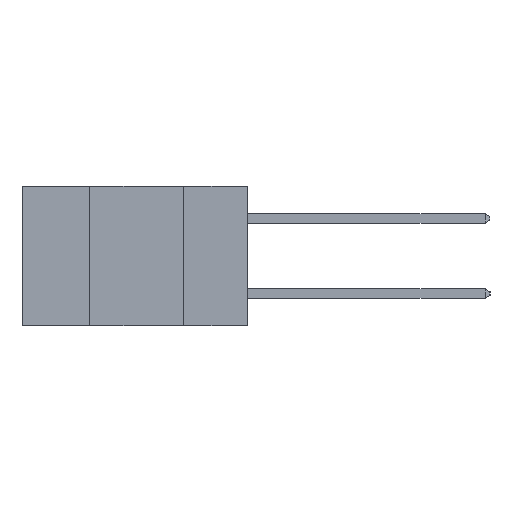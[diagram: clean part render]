
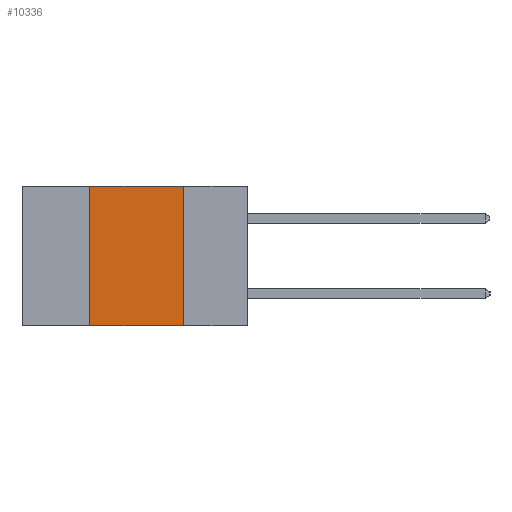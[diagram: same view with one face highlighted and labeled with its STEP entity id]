
A CAD part, left-side view. The second image highlights one B-rep face of the part: STEP entity #10336.
In plain terms, the highlighted planar face has unit normal (-1, 0, 0).
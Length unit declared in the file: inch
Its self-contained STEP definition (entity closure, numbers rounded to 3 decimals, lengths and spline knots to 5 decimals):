
#260 = CARTESIAN_POINT ( 'NONE',  ( 0., 0.6, 0. ) ) ;
#1166 = VERTEX_POINT ( 'NONE', #12505 ) ;
#1240 = CARTESIAN_POINT ( 'NONE',  ( 0., 0.6, -0.37 ) ) ;
#2592 = CARTESIAN_POINT ( 'NONE',  ( 0., 0.42, -0.37 ) ) ;
#3094 = CARTESIAN_POINT ( 'NONE',  ( 0., 0.17, -0.37 ) ) ;
#3342 = LINE ( 'NONE', #260, #7671 ) ;
#3726 = DIRECTION ( 'NONE',  ( 0., 0., -1. ) ) ;
#5409 = VECTOR ( 'NONE', #6455, 39.37008 ) ;
#5919 = LINE ( 'NONE', #17534, #5409 ) ;
#6112 = CARTESIAN_POINT ( 'NONE',  ( 0., 0.42, 0. ) ) ;
#6242 = FACE_OUTER_BOUND ( 'NONE', #17849, .T. ) ;
#6376 = DIRECTION ( 'NONE',  ( 0., 0., -1. ) ) ;
#6455 = DIRECTION ( 'NONE',  ( 0., 0., 1. ) ) ;
#7671 = VECTOR ( 'NONE', #11503, 39.37008 ) ;
#7722 = ORIENTED_EDGE ( 'NONE', *, *, #11898, .F. ) ;
#7904 = VERTEX_POINT ( 'NONE', #2592 ) ;
#8042 = EDGE_CURVE ( 'NONE', #11130, #1166, #16071, .T. ) ;
#10136 = PLANE ( 'NONE',  #19233 ) ;
#10336 = ADVANCED_FACE ( 'NONE', ( #6242 ), #10136, .F. ) ;
#10875 = DIRECTION ( 'NONE',  ( 0., -1., 0. ) ) ;
#10912 = ORIENTED_EDGE ( 'NONE', *, *, #17921, .F. ) ;
#11130 = VERTEX_POINT ( 'NONE', #14127 ) ;
#11503 = DIRECTION ( 'NONE',  ( 0., -1., 0. ) ) ;
#11642 = CARTESIAN_POINT ( 'NONE',  ( 0., 0.6, 0. ) ) ;
#11898 = EDGE_CURVE ( 'NONE', #7904, #15454, #5919, .T. ) ;
#12290 = VECTOR ( 'NONE', #10875, 39.37008 ) ;
#12505 = CARTESIAN_POINT ( 'NONE',  ( 0., 0.17, -0.37 ) ) ;
#13328 = DIRECTION ( 'NONE',  ( 1., 0., 0. ) ) ;
#14127 = CARTESIAN_POINT ( 'NONE',  ( 0., 0.17, 0. ) ) ;
#14188 = ORIENTED_EDGE ( 'NONE', *, *, #19579, .T. ) ;
#15454 = VERTEX_POINT ( 'NONE', #6112 ) ;
#15606 = VECTOR ( 'NONE', #6376, 39.37008 ) ;
#15642 = ORIENTED_EDGE ( 'NONE', *, *, #8042, .F. ) ;
#16071 = LINE ( 'NONE', #3094, #15606 ) ;
#17534 = CARTESIAN_POINT ( 'NONE',  ( 0., 0.42, -0.37 ) ) ;
#17849 = EDGE_LOOP ( 'NONE', ( #15642, #10912, #7722, #14188 ) ) ;
#17921 = EDGE_CURVE ( 'NONE', #15454, #11130, #3342, .T. ) ;
#19233 = AXIS2_PLACEMENT_3D ( 'NONE', #11642, #13328, #3726 ) ;
#19579 = EDGE_CURVE ( 'NONE', #7904, #1166, #20509, .T. ) ;
#20509 = LINE ( 'NONE', #1240, #12290 ) ;
